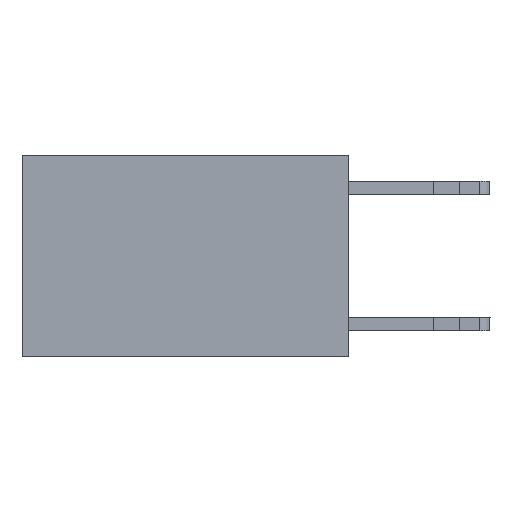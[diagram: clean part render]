
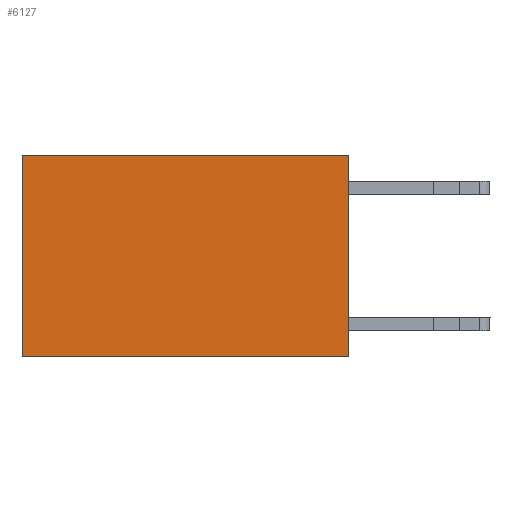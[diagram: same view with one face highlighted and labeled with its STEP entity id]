
A CAD part, left-side view. The second image highlights one B-rep face of the part: STEP entity #6127.
In plain terms, the highlighted planar face has unit normal (-1, 0, 0).
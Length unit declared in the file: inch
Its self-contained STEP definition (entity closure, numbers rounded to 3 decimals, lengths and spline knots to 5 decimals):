
#288 = CARTESIAN_POINT ( 'NONE',  ( 0.2625, 0.6, -0.37 ) ) ;
#549 = AXIS2_PLACEMENT_3D ( 'NONE', #6927, #648, #9464 ) ;
#648 = DIRECTION ( 'NONE',  ( 1., 0., 0. ) ) ;
#781 = DIRECTION ( 'NONE',  ( 0., 1., 0. ) ) ;
#892 = CARTESIAN_POINT ( 'NONE',  ( 0.2625, 0.6, 0. ) ) ;
#3211 = ORIENTED_EDGE ( 'NONE', *, *, #12046, .T. ) ;
#3640 = VERTEX_POINT ( 'NONE', #892 ) ;
#4418 = ORIENTED_EDGE ( 'NONE', *, *, #15446, .F. ) ;
#4677 = VERTEX_POINT ( 'NONE', #288 ) ;
#4870 = LINE ( 'NONE', #5264, #10340 ) ;
#5264 = CARTESIAN_POINT ( 'NONE',  ( 0.2625, 0., 0. ) ) ;
#5363 = VERTEX_POINT ( 'NONE', #11473 ) ;
#5661 = EDGE_CURVE ( 'NONE', #5363, #14950, #7143, .T. ) ;
#5933 = ORIENTED_EDGE ( 'NONE', *, *, #15132, .T. ) ;
#6023 = LINE ( 'NONE', #10828, #8964 ) ;
#6127 = ADVANCED_FACE ( 'NONE', ( #8641 ), #15606, .F. ) ;
#6306 = CARTESIAN_POINT ( 'NONE',  ( 0.2625, 0.6, 0. ) ) ;
#6742 = VECTOR ( 'NONE', #7108, 39.37008 ) ;
#6927 = CARTESIAN_POINT ( 'NONE',  ( 0.2625, 0., 0. ) ) ;
#7108 = DIRECTION ( 'NONE',  ( 0., 0., -1. ) ) ;
#7143 = LINE ( 'NONE', #12086, #6742 ) ;
#7394 = CARTESIAN_POINT ( 'NONE',  ( 0.2625, 0., -0.37 ) ) ;
#8111 = EDGE_LOOP ( 'NONE', ( #3211, #4418, #12773, #5933 ) ) ;
#8641 = FACE_OUTER_BOUND ( 'NONE', #8111, .T. ) ;
#8964 = VECTOR ( 'NONE', #781, 39.37008 ) ;
#9033 = DIRECTION ( 'NONE',  ( 0., 1., 0. ) ) ;
#9446 = VECTOR ( 'NONE', #14980, 39.37008 ) ;
#9464 = DIRECTION ( 'NONE',  ( 0., 0., -1. ) ) ;
#10340 = VECTOR ( 'NONE', #9033, 39.37008 ) ;
#10828 = CARTESIAN_POINT ( 'NONE',  ( 0.2625, 0., -0.37 ) ) ;
#11473 = CARTESIAN_POINT ( 'NONE',  ( 0.2625, 0., 0. ) ) ;
#12046 = EDGE_CURVE ( 'NONE', #3640, #4677, #15615, .T. ) ;
#12086 = CARTESIAN_POINT ( 'NONE',  ( 0.2625, 0., 0. ) ) ;
#12773 = ORIENTED_EDGE ( 'NONE', *, *, #5661, .F. ) ;
#14950 = VERTEX_POINT ( 'NONE', #7394 ) ;
#14980 = DIRECTION ( 'NONE',  ( 0., 0., -1. ) ) ;
#15132 = EDGE_CURVE ( 'NONE', #5363, #3640, #4870, .T. ) ;
#15446 = EDGE_CURVE ( 'NONE', #14950, #4677, #6023, .T. ) ;
#15606 = PLANE ( 'NONE',  #549 ) ;
#15615 = LINE ( 'NONE', #6306, #9446 ) ;
